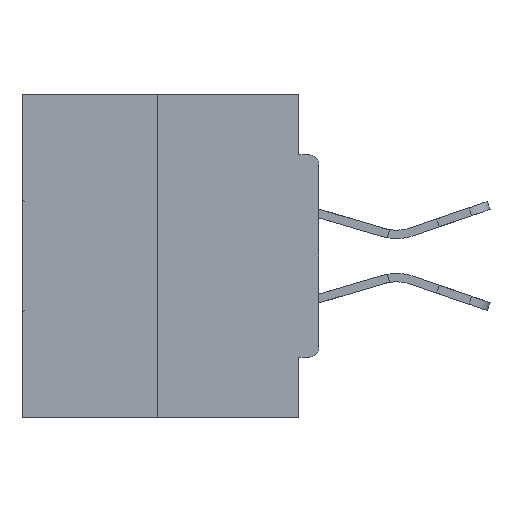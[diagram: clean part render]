
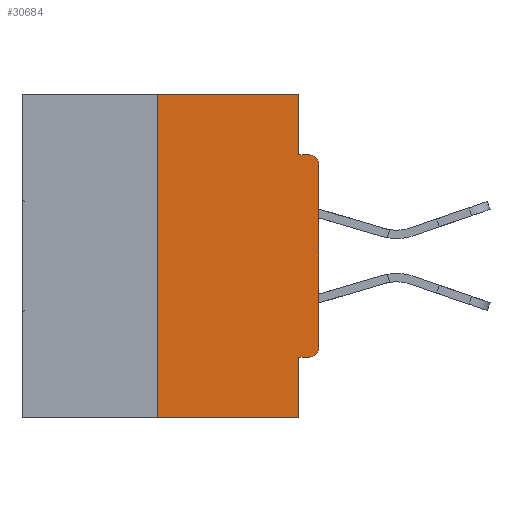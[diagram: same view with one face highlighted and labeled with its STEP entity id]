
A CAD part, left-side view. The second image highlights one B-rep face of the part: STEP entity #30684.
In plain terms, the highlighted planar face has unit normal (-1, 0, 0).
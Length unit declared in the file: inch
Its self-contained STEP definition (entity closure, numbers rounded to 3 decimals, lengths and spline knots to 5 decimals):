
#1599 = VECTOR ( 'NONE', #4418, 39.37008 ) ;
#2980 = CARTESIAN_POINT ( 'NONE',  ( 0., 0., -0.0935 ) ) ;
#3596 = ORIENTED_EDGE ( 'NONE', *, *, #23803, .F. ) ;
#3671 = VERTEX_POINT ( 'NONE', #17710 ) ;
#3765 = CARTESIAN_POINT ( 'NONE',  ( 0., 0., -0.3915 ) ) ;
#3797 = AXIS2_PLACEMENT_3D ( 'NONE', #5834, #12336, #18862 ) ;
#3943 = FACE_OUTER_BOUND ( 'NONE', #15433, .T. ) ;
#4418 = DIRECTION ( 'NONE',  ( 0., 0., 1. ) ) ;
#4464 = CIRCLE ( 'NONE', #3797, 0.015 ) ;
#4760 = EDGE_CURVE ( 'NONE', #41523, #15131, #19807, .T. ) ;
#5834 = CARTESIAN_POINT ( 'NONE',  ( 0., 0.015, -0.1085 ) ) ;
#6951 = CARTESIAN_POINT ( 'NONE',  ( 0., 0.031, 0. ) ) ;
#7071 = EDGE_CURVE ( 'NONE', #36905, #40166, #23856, .T. ) ;
#7590 = LINE ( 'NONE', #10935, #1599 ) ;
#8005 = ORIENTED_EDGE ( 'NONE', *, *, #39229, .T. ) ;
#8272 = LINE ( 'NONE', #39934, #15505 ) ;
#9066 = AXIS2_PLACEMENT_3D ( 'NONE', #19384, #13484, #26410 ) ;
#10935 = CARTESIAN_POINT ( 'NONE',  ( 0., 0., 0. ) ) ;
#12336 = DIRECTION ( 'NONE',  ( -1., 0., 0. ) ) ;
#12675 = ORIENTED_EDGE ( 'NONE', *, *, #16692, .T. ) ;
#13214 = EDGE_CURVE ( 'NONE', #13376, #3671, #30702, .T. ) ;
#13376 = VERTEX_POINT ( 'NONE', #20002 ) ;
#13484 = DIRECTION ( 'NONE',  ( -1., 0., 0. ) ) ;
#13612 = PLANE ( 'NONE',  #20606 ) ;
#14006 = VERTEX_POINT ( 'NONE', #27978 ) ;
#15131 = VERTEX_POINT ( 'NONE', #3765 ) ;
#15433 = EDGE_LOOP ( 'NONE', ( #3596, #36326, #12675, #27098, #24272, #33591, #8005, #20162, #25626, #19340 ) ) ;
#15505 = VECTOR ( 'NONE', #24286, 39.37008 ) ;
#16221 = CARTESIAN_POINT ( 'NONE',  ( 0., 0.015, -0.4065 ) ) ;
#16692 = EDGE_CURVE ( 'NONE', #13376, #14006, #37193, .T. ) ;
#17710 = CARTESIAN_POINT ( 'NONE',  ( 0., 0.25, 0. ) ) ;
#18862 = DIRECTION ( 'NONE',  ( 0., 0., -1. ) ) ;
#19340 = ORIENTED_EDGE ( 'NONE', *, *, #39148, .F. ) ;
#19384 = CARTESIAN_POINT ( 'NONE',  ( 0., 0.015, -0.3915 ) ) ;
#19807 = CIRCLE ( 'NONE', #9066, 0.015 ) ;
#19940 = DIRECTION ( 'NONE',  ( 0., 0., -1. ) ) ;
#20002 = CARTESIAN_POINT ( 'NONE',  ( 0., 0.25, -0.5 ) ) ;
#20162 = ORIENTED_EDGE ( 'NONE', *, *, #32479, .T. ) ;
#20606 = AXIS2_PLACEMENT_3D ( 'NONE', #38772, #34631, #19940 ) ;
#21493 = EDGE_CURVE ( 'NONE', #41523, #28004, #8272, .T. ) ;
#23225 = CARTESIAN_POINT ( 'NONE',  ( 0., 0.031, -0.5 ) ) ;
#23315 = EDGE_CURVE ( 'NONE', #28004, #14006, #29570, .T. ) ;
#23803 = EDGE_CURVE ( 'NONE', #3671, #28431, #36598, .T. ) ;
#23856 = LINE ( 'NONE', #2980, #33214 ) ;
#24272 = ORIENTED_EDGE ( 'NONE', *, *, #21493, .F. ) ;
#24286 = DIRECTION ( 'NONE',  ( 0., 1., 0. ) ) ;
#25626 = ORIENTED_EDGE ( 'NONE', *, *, #7071, .F. ) ;
#26410 = DIRECTION ( 'NONE',  ( 0., 0., -1. ) ) ;
#26789 = VECTOR ( 'NONE', #30469, 39.37008 ) ;
#27098 = ORIENTED_EDGE ( 'NONE', *, *, #23315, .F. ) ;
#27477 = CARTESIAN_POINT ( 'NONE',  ( 0., 0.46, -0.5 ) ) ;
#27974 = CARTESIAN_POINT ( 'NONE',  ( 0., 0.031, -0.0935 ) ) ;
#27978 = CARTESIAN_POINT ( 'NONE',  ( 0., 0.031, -0.5 ) ) ;
#28004 = VERTEX_POINT ( 'NONE', #32735 ) ;
#28020 = CARTESIAN_POINT ( 'NONE',  ( 0., 0.015, -0.0935 ) ) ;
#28431 = VERTEX_POINT ( 'NONE', #6951 ) ;
#28821 = VECTOR ( 'NONE', #40347, 39.37008 ) ;
#29570 = LINE ( 'NONE', #23225, #34869 ) ;
#29948 = DIRECTION ( 'NONE',  ( 0., 0., -1. ) ) ;
#30469 = DIRECTION ( 'NONE',  ( 0., -1., 0. ) ) ;
#30489 = DIRECTION ( 'NONE',  ( 0., 0., 1. ) ) ;
#30684 = ADVANCED_FACE ( 'NONE', ( #3943 ), #13612, .F. ) ;
#30702 = LINE ( 'NONE', #34842, #33156 ) ;
#32249 = VERTEX_POINT ( 'NONE', #38830 ) ;
#32479 = EDGE_CURVE ( 'NONE', #32249, #40166, #4464, .T. ) ;
#32735 = CARTESIAN_POINT ( 'NONE',  ( 0., 0.031, -0.4065 ) ) ;
#32958 = DIRECTION ( 'NONE',  ( 0., 0., -1. ) ) ;
#33005 = CARTESIAN_POINT ( 'NONE',  ( 0., 0.46, 0. ) ) ;
#33156 = VECTOR ( 'NONE', #30489, 39.37008 ) ;
#33214 = VECTOR ( 'NONE', #40777, 39.37008 ) ;
#33591 = ORIENTED_EDGE ( 'NONE', *, *, #4760, .T. ) ;
#34613 = VECTOR ( 'NONE', #29948, 39.37008 ) ;
#34631 = DIRECTION ( 'NONE',  ( 1., 0., 0. ) ) ;
#34842 = CARTESIAN_POINT ( 'NONE',  ( 0., 0.25, 0. ) ) ;
#34869 = VECTOR ( 'NONE', #32958, 39.37008 ) ;
#36326 = ORIENTED_EDGE ( 'NONE', *, *, #13214, .F. ) ;
#36598 = LINE ( 'NONE', #33005, #26789 ) ;
#36905 = VERTEX_POINT ( 'NONE', #27974 ) ;
#37135 = LINE ( 'NONE', #39879, #34613 ) ;
#37193 = LINE ( 'NONE', #27477, #28821 ) ;
#38772 = CARTESIAN_POINT ( 'NONE',  ( 0., 0.46, 0. ) ) ;
#38830 = CARTESIAN_POINT ( 'NONE',  ( 0., 0., -0.1085 ) ) ;
#39148 = EDGE_CURVE ( 'NONE', #28431, #36905, #37135, .T. ) ;
#39229 = EDGE_CURVE ( 'NONE', #15131, #32249, #7590, .T. ) ;
#39879 = CARTESIAN_POINT ( 'NONE',  ( 0., 0.031, 0. ) ) ;
#39934 = CARTESIAN_POINT ( 'NONE',  ( 0., 0., -0.4065 ) ) ;
#40166 = VERTEX_POINT ( 'NONE', #28020 ) ;
#40347 = DIRECTION ( 'NONE',  ( 0., -1., 0. ) ) ;
#40777 = DIRECTION ( 'NONE',  ( 0., -1., 0. ) ) ;
#41523 = VERTEX_POINT ( 'NONE', #16221 ) ;
